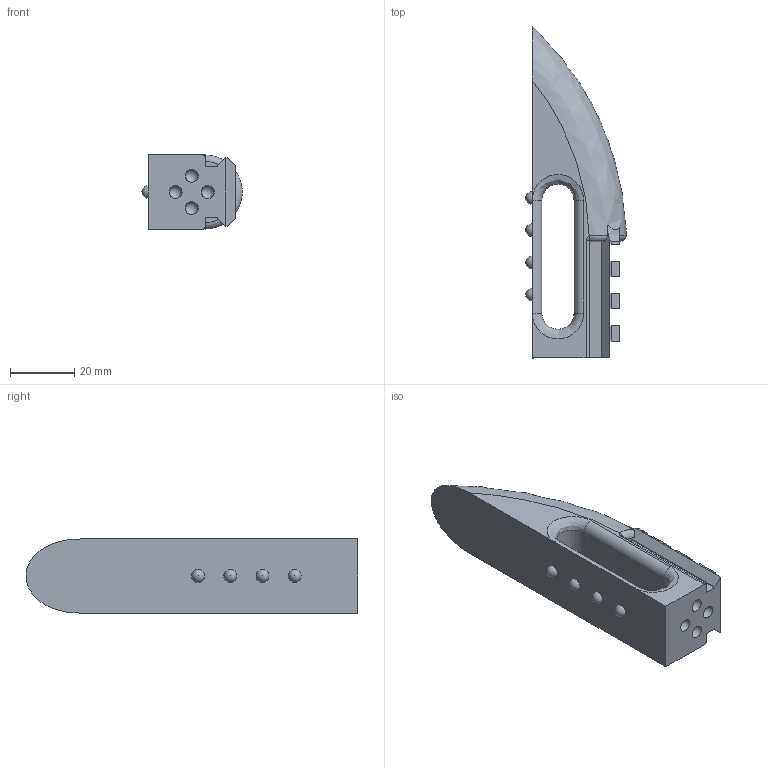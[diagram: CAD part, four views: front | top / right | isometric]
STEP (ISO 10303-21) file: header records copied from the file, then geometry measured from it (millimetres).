
FILE_DESCRIPTION (( 'STEP AP214' ), '1' );
FILE_NAME ('Stock_Rail_Front_V2.step', '2016-01-25T18:17:28', ( 'WarFairy' ), ( '' ), 'SwSTEP 2.0', 'SolidWorks 2015', '' );
FILE_SCHEMA (( 'AUTOMOTIVE_DESIGN' ));
Length unit declared in the file: millimetre
Products named in the file (1): Stock_Rail_Front_V2
Bounding box: 31.2 x 103.07 x 23.02 mm (x, y, z)
Volume: 36292.4 mm3; surface area: 11106.9 mm2
Topology: 1 solids, 1 shells, 72 faces, 212 edges, 134 vertices
Faces by surface type: plane 42, bspline 14, cylinder 8, sphere 8
Entity records: 2954 total; most frequent: CARTESIAN_POINT 1277, ORIENTED_EDGE 372, DIRECTION 285, EDGE_CURVE 186, VERTEX_POINT 122, LINE 119, VECTOR 119, AXIS2_PLACEMENT_3D 83
